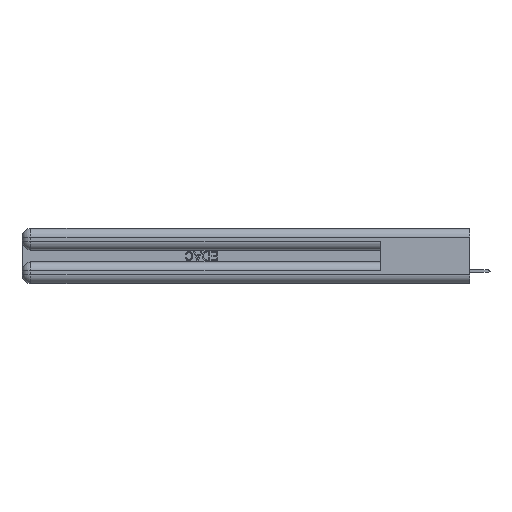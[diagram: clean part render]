
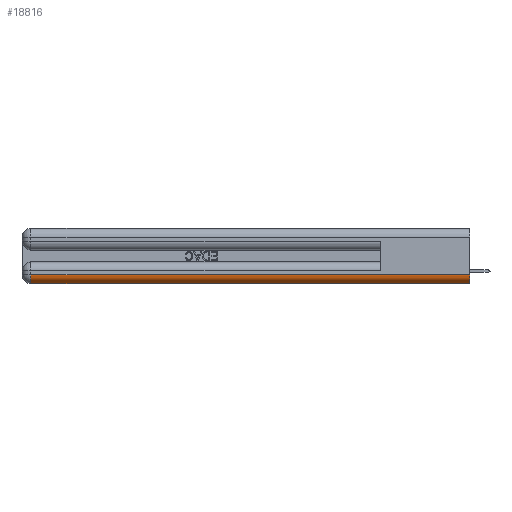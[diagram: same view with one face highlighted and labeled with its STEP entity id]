
A CAD part, left-side view. The second image highlights one B-rep face of the part: STEP entity #18816.
In plain terms, the highlighted cylindrical face has radius 1.524 mm (diameter 3.048 mm), a partial arc.
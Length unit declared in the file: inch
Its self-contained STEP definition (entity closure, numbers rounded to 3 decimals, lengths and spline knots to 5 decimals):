
#2085 = VERTEX_POINT ( 'NONE', #20368 ) ;
#6115 = DIRECTION ( 'NONE',  ( 0., -1., 0. ) ) ;
#7161 = AXIS2_PLACEMENT_3D ( 'NONE', #23831, #6115, #41101 ) ;
#7416 = VERTEX_POINT ( 'NONE', #16569 ) ;
#8732 = VERTEX_POINT ( 'NONE', #34735 ) ;
#8768 = AXIS2_PLACEMENT_3D ( 'NONE', #12811, #19846, #9393 ) ;
#8948 = CYLINDRICAL_SURFACE ( 'NONE', #8768, 0.06 ) ;
#9393 = DIRECTION ( 'NONE',  ( 0., 0., 1. ) ) ;
#10278 = CARTESIAN_POINT ( 'NONE',  ( 0.06, 2.94, 0. ) ) ;
#12811 = CARTESIAN_POINT ( 'NONE',  ( 0.06, 0., 0.06 ) ) ;
#14161 = CARTESIAN_POINT ( 'NONE',  ( 0.06, 2.94, 0.06 ) ) ;
#14211 = EDGE_CURVE ( 'NONE', #8732, #7416, #21685, .T. ) ;
#16569 = CARTESIAN_POINT ( 'NONE',  ( 0.06, 0., 0. ) ) ;
#18816 = ADVANCED_FACE ( 'NONE', ( #25328 ), #8948, .T. ) ;
#19846 = DIRECTION ( 'NONE',  ( 0., 1., 0. ) ) ;
#20368 = CARTESIAN_POINT ( 'NONE',  ( 0., 2.94, 0.06 ) ) ;
#20947 = CARTESIAN_POINT ( 'NONE',  ( 0., 0., 0.06 ) ) ;
#21685 = CIRCLE ( 'NONE', #7161, 0.06 ) ;
#21720 = AXIS2_PLACEMENT_3D ( 'NONE', #14161, #31202, #42092 ) ;
#22968 = EDGE_CURVE ( 'NONE', #2085, #8732, #37758, .T. ) ;
#23831 = CARTESIAN_POINT ( 'NONE',  ( 0.06, 0., 0.06 ) ) ;
#24139 = DIRECTION ( 'NONE',  ( 0., -1., 0. ) ) ;
#25328 = FACE_OUTER_BOUND ( 'NONE', #37734, .T. ) ;
#26118 = ORIENTED_EDGE ( 'NONE', *, *, #22968, .F. ) ;
#27009 = ORIENTED_EDGE ( 'NONE', *, *, #14211, .F. ) ;
#30296 = LINE ( 'NONE', #30741, #37467 ) ;
#30516 = EDGE_CURVE ( 'NONE', #7416, #44728, #30296, .T. ) ;
#30741 = CARTESIAN_POINT ( 'NONE',  ( 0.06, 3., 0. ) ) ;
#31202 = DIRECTION ( 'NONE',  ( 0., 1., 0. ) ) ;
#31549 = ORIENTED_EDGE ( 'NONE', *, *, #35805, .F. ) ;
#34735 = CARTESIAN_POINT ( 'NONE',  ( 0., 0., 0.06 ) ) ;
#35173 = VECTOR ( 'NONE', #24139, 39.37008 ) ;
#35805 = EDGE_CURVE ( 'NONE', #44728, #2085, #42019, .T. ) ;
#37467 = VECTOR ( 'NONE', #44148, 39.37008 ) ;
#37528 = ORIENTED_EDGE ( 'NONE', *, *, #30516, .F. ) ;
#37734 = EDGE_LOOP ( 'NONE', ( #27009, #26118, #31549, #37528 ) ) ;
#37758 = LINE ( 'NONE', #20947, #35173 ) ;
#41101 = DIRECTION ( 'NONE',  ( 0., 0., 1. ) ) ;
#42019 = CIRCLE ( 'NONE', #21720, 0.06 ) ;
#42092 = DIRECTION ( 'NONE',  ( 0., 0., 1. ) ) ;
#44148 = DIRECTION ( 'NONE',  ( 0., 1., 0. ) ) ;
#44728 = VERTEX_POINT ( 'NONE', #10278 ) ;
